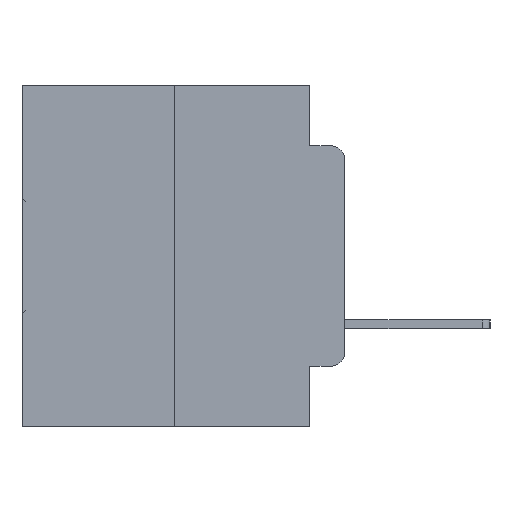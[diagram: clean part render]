
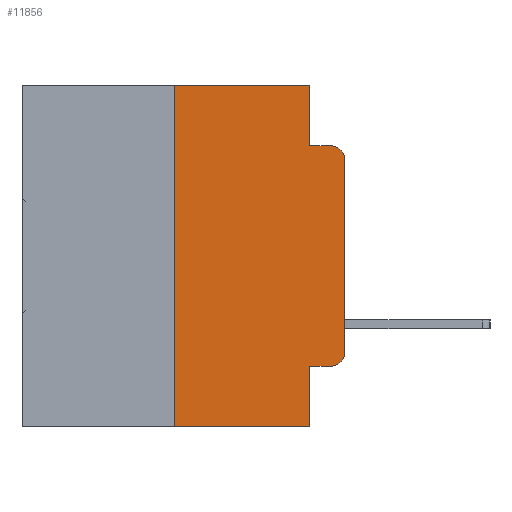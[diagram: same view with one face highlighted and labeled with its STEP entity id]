
A CAD part, left-side view. The second image highlights one B-rep face of the part: STEP entity #11856.
In plain terms, the highlighted planar face has unit normal (-1, 0, 0).
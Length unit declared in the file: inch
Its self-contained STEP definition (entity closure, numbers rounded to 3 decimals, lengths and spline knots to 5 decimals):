
#409 = VERTEX_POINT ( 'NONE', #15911 ) ;
#1360 = DIRECTION ( 'NONE',  ( 0., -1., 0. ) ) ;
#1787 = EDGE_CURVE ( 'NONE', #3331, #19405, #12877, .T. ) ;
#2027 = CARTESIAN_POINT ( 'NONE',  ( 0., 0.25, -0.5 ) ) ;
#2083 = LINE ( 'NONE', #13690, #2860 ) ;
#2860 = VECTOR ( 'NONE', #27746, 39.37008 ) ;
#3268 = CARTESIAN_POINT ( 'NONE',  ( 0., 0.051, -0.5 ) ) ;
#3331 = VERTEX_POINT ( 'NONE', #29349 ) ;
#3731 = ORIENTED_EDGE ( 'NONE', *, *, #23022, .T. ) ;
#3762 = ORIENTED_EDGE ( 'NONE', *, *, #4435, .T. ) ;
#3801 = LINE ( 'NONE', #6041, #21545 ) ;
#3991 = VERTEX_POINT ( 'NONE', #3268 ) ;
#4068 = EDGE_CURVE ( 'NONE', #409, #3991, #3801, .T. ) ;
#4412 = AXIS2_PLACEMENT_3D ( 'NONE', #22190, #7860, #24588 ) ;
#4435 = EDGE_CURVE ( 'NONE', #19405, #4933, #4536, .T. ) ;
#4536 = CIRCLE ( 'NONE', #7682, 0.02 ) ;
#4769 = CARTESIAN_POINT ( 'NONE',  ( 0., 0.051, -0.0885 ) ) ;
#4933 = VERTEX_POINT ( 'NONE', #7494 ) ;
#5221 = VECTOR ( 'NONE', #24301, 39.37008 ) ;
#5263 = ORIENTED_EDGE ( 'NONE', *, *, #4068, .F. ) ;
#5507 = DIRECTION ( 'NONE',  ( 0., 0., -1. ) ) ;
#5647 = VERTEX_POINT ( 'NONE', #19690 ) ;
#5860 = EDGE_CURVE ( 'NONE', #5647, #30232, #23652, .T. ) ;
#6041 = CARTESIAN_POINT ( 'NONE',  ( 0., 0.051, 0. ) ) ;
#6365 = CARTESIAN_POINT ( 'NONE',  ( 0., 0., 0. ) ) ;
#6381 = CARTESIAN_POINT ( 'NONE',  ( 0., 0.25, 0. ) ) ;
#7405 = VECTOR ( 'NONE', #9708, 39.37008 ) ;
#7494 = CARTESIAN_POINT ( 'NONE',  ( 0., 0.02, -0.0885 ) ) ;
#7536 = CARTESIAN_POINT ( 'NONE',  ( 0., 0.051, 0. ) ) ;
#7682 = AXIS2_PLACEMENT_3D ( 'NONE', #24694, #10410, #27054 ) ;
#7860 = DIRECTION ( 'NONE',  ( -1., 0., 0. ) ) ;
#8280 = VERTEX_POINT ( 'NONE', #2027 ) ;
#9445 = DIRECTION ( 'NONE',  ( 0., -1., 0. ) ) ;
#9708 = DIRECTION ( 'NONE',  ( 0., 0., 1. ) ) ;
#10317 = EDGE_LOOP ( 'NONE', ( #21502, #3762, #17823, #12151, #20019, #27734, #3731, #5263, #18203, #25923 ) ) ;
#10332 = PLANE ( 'NONE',  #11553 ) ;
#10410 = DIRECTION ( 'NONE',  ( -1., 0., 0. ) ) ;
#11553 = AXIS2_PLACEMENT_3D ( 'NONE', #12779, #19987, #5507 ) ;
#11856 = ADVANCED_FACE ( 'NONE', ( #25898 ), #10332, .F. ) ;
#12151 = ORIENTED_EDGE ( 'NONE', *, *, #5860, .F. ) ;
#12657 = VERTEX_POINT ( 'NONE', #27640 ) ;
#12779 = CARTESIAN_POINT ( 'NONE',  ( 0., 0.473, 0. ) ) ;
#12877 = LINE ( 'NONE', #6365, #13633 ) ;
#13202 = DIRECTION ( 'NONE',  ( 0., -1., 0. ) ) ;
#13556 = CARTESIAN_POINT ( 'NONE',  ( 0., 0.051, -0.0885 ) ) ;
#13633 = VECTOR ( 'NONE', #25220, 39.37008 ) ;
#13690 = CARTESIAN_POINT ( 'NONE',  ( 0., 0.473, -0.5 ) ) ;
#13898 = LINE ( 'NONE', #30933, #7405 ) ;
#15741 = DIRECTION ( 'NONE',  ( 0., 0., -1. ) ) ;
#15911 = CARTESIAN_POINT ( 'NONE',  ( 0., 0.051, -0.4115 ) ) ;
#17823 = ORIENTED_EDGE ( 'NONE', *, *, #23620, .F. ) ;
#18110 = VERTEX_POINT ( 'NONE', #6381 ) ;
#18203 = ORIENTED_EDGE ( 'NONE', *, *, #29532, .T. ) ;
#18298 = EDGE_CURVE ( 'NONE', #8280, #18110, #13898, .T. ) ;
#19405 = VERTEX_POINT ( 'NONE', #30659 ) ;
#19690 = CARTESIAN_POINT ( 'NONE',  ( 0., 0.051, 0. ) ) ;
#19987 = DIRECTION ( 'NONE',  ( 1., 0., 0. ) ) ;
#20019 = ORIENTED_EDGE ( 'NONE', *, *, #30487, .F. ) ;
#21372 = VECTOR ( 'NONE', #13202, 39.37008 ) ;
#21502 = ORIENTED_EDGE ( 'NONE', *, *, #1787, .T. ) ;
#21545 = VECTOR ( 'NONE', #15741, 39.37008 ) ;
#21663 = EDGE_CURVE ( 'NONE', #12657, #3331, #29173, .T. ) ;
#22190 = CARTESIAN_POINT ( 'NONE',  ( 0., 0.02, -0.3915 ) ) ;
#22849 = LINE ( 'NONE', #13556, #28362 ) ;
#23022 = EDGE_CURVE ( 'NONE', #8280, #3991, #2083, .T. ) ;
#23620 = EDGE_CURVE ( 'NONE', #30232, #4933, #22849, .T. ) ;
#23652 = LINE ( 'NONE', #7536, #5221 ) ;
#23742 = CARTESIAN_POINT ( 'NONE',  ( 0., 0.051, -0.4115 ) ) ;
#24301 = DIRECTION ( 'NONE',  ( 0., 0., -1. ) ) ;
#24588 = DIRECTION ( 'NONE',  ( 0., 0., -1. ) ) ;
#24694 = CARTESIAN_POINT ( 'NONE',  ( 0., 0.02, -0.1085 ) ) ;
#25019 = CARTESIAN_POINT ( 'NONE',  ( 0., 0.473, 0. ) ) ;
#25134 = LINE ( 'NONE', #23742, #25886 ) ;
#25220 = DIRECTION ( 'NONE',  ( 0., 0., 1. ) ) ;
#25886 = VECTOR ( 'NONE', #9445, 39.37008 ) ;
#25898 = FACE_OUTER_BOUND ( 'NONE', #10317, .T. ) ;
#25923 = ORIENTED_EDGE ( 'NONE', *, *, #21663, .T. ) ;
#27054 = DIRECTION ( 'NONE',  ( 0., 0., -1. ) ) ;
#27640 = CARTESIAN_POINT ( 'NONE',  ( 0., 0.02, -0.4115 ) ) ;
#27649 = LINE ( 'NONE', #25019, #21372 ) ;
#27734 = ORIENTED_EDGE ( 'NONE', *, *, #18298, .F. ) ;
#27746 = DIRECTION ( 'NONE',  ( 0., -1., 0. ) ) ;
#28362 = VECTOR ( 'NONE', #1360, 39.37008 ) ;
#29173 = CIRCLE ( 'NONE', #4412, 0.02 ) ;
#29349 = CARTESIAN_POINT ( 'NONE',  ( 0., 0., -0.3915 ) ) ;
#29532 = EDGE_CURVE ( 'NONE', #409, #12657, #25134, .T. ) ;
#30232 = VERTEX_POINT ( 'NONE', #4769 ) ;
#30487 = EDGE_CURVE ( 'NONE', #18110, #5647, #27649, .T. ) ;
#30659 = CARTESIAN_POINT ( 'NONE',  ( 0., 0., -0.1085 ) ) ;
#30933 = CARTESIAN_POINT ( 'NONE',  ( 0., 0.25, 0. ) ) ;
